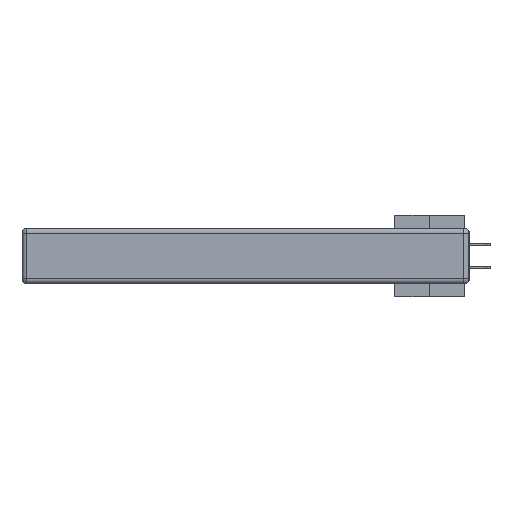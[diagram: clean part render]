
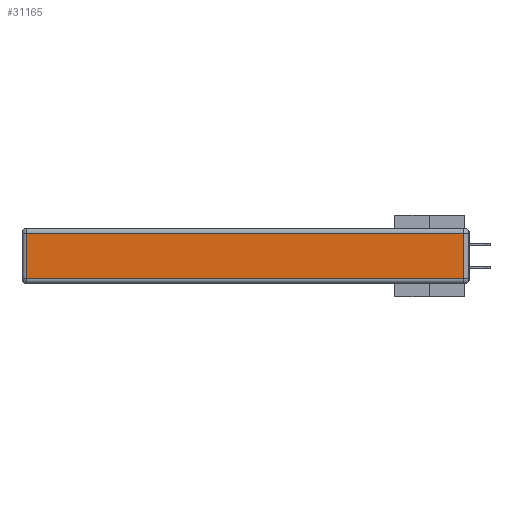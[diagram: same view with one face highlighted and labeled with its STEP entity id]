
A CAD part, left-side view. The second image highlights one B-rep face of the part: STEP entity #31165.
In plain terms, the highlighted planar face has unit normal (-1, 0, 0).
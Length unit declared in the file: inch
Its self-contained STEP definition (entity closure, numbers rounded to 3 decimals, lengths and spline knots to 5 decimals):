
#461 = ORIENTED_EDGE ( 'NONE', *, *, #7113, .T. ) ;
#4865 = VERTEX_POINT ( 'NONE', #38495 ) ;
#5474 = CARTESIAN_POINT ( 'NONE',  ( 0., 2.75, -0.03 ) ) ;
#6010 = DIRECTION ( 'NONE',  ( 0., 0., 1. ) ) ;
#7113 = EDGE_CURVE ( 'NONE', #35463, #4865, #17173, .T. ) ;
#7838 = CARTESIAN_POINT ( 'NONE',  ( 0., 0.03, -0.313 ) ) ;
#9861 = EDGE_CURVE ( 'NONE', #18128, #13395, #24023, .T. ) ;
#11169 = CARTESIAN_POINT ( 'NONE',  ( 0., 2.72, -0.313 ) ) ;
#11842 = DIRECTION ( 'NONE',  ( 0., 0., -1. ) ) ;
#12376 = LINE ( 'NONE', #33854, #29495 ) ;
#13394 = AXIS2_PLACEMENT_3D ( 'NONE', #35403, #17165, #38441 ) ;
#13395 = VERTEX_POINT ( 'NONE', #7838 ) ;
#14112 = PLANE ( 'NONE',  #13394 ) ;
#14118 = ORIENTED_EDGE ( 'NONE', *, *, #27537, .T. ) ;
#14426 = ORIENTED_EDGE ( 'NONE', *, *, #9861, .T. ) ;
#15076 = ORIENTED_EDGE ( 'NONE', *, *, #37503, .T. ) ;
#17165 = DIRECTION ( 'NONE',  ( -1., 0., 0. ) ) ;
#17173 = LINE ( 'NONE', #5474, #18146 ) ;
#18128 = VERTEX_POINT ( 'NONE', #11169 ) ;
#18146 = VECTOR ( 'NONE', #39061, 39.37008 ) ;
#20737 = LINE ( 'NONE', #24477, #35981 ) ;
#24023 = LINE ( 'NONE', #38869, #34996 ) ;
#24477 = CARTESIAN_POINT ( 'NONE',  ( 0., 2.72, -0.343 ) ) ;
#24959 = EDGE_LOOP ( 'NONE', ( #14426, #15076, #461, #14118 ) ) ;
#27537 = EDGE_CURVE ( 'NONE', #4865, #18128, #20737, .T. ) ;
#29495 = VECTOR ( 'NONE', #6010, 39.37008 ) ;
#31165 = ADVANCED_FACE ( 'NONE', ( #31458 ), #14112, .T. ) ;
#31458 = FACE_OUTER_BOUND ( 'NONE', #24959, .T. ) ;
#32611 = DIRECTION ( 'NONE',  ( 0., -1., 0. ) ) ;
#33854 = CARTESIAN_POINT ( 'NONE',  ( 0., 0.03, -0.343 ) ) ;
#34996 = VECTOR ( 'NONE', #32611, 39.37008 ) ;
#35403 = CARTESIAN_POINT ( 'NONE',  ( 0., 0., -0.343 ) ) ;
#35463 = VERTEX_POINT ( 'NONE', #36331 ) ;
#35981 = VECTOR ( 'NONE', #11842, 39.37008 ) ;
#36331 = CARTESIAN_POINT ( 'NONE',  ( 0., 0.03, -0.03 ) ) ;
#37503 = EDGE_CURVE ( 'NONE', #13395, #35463, #12376, .T. ) ;
#38441 = DIRECTION ( 'NONE',  ( 0., 0., 1. ) ) ;
#38495 = CARTESIAN_POINT ( 'NONE',  ( 0., 2.72, -0.03 ) ) ;
#38869 = CARTESIAN_POINT ( 'NONE',  ( 0., 0., -0.313 ) ) ;
#39061 = DIRECTION ( 'NONE',  ( 0., 1., 0. ) ) ;
